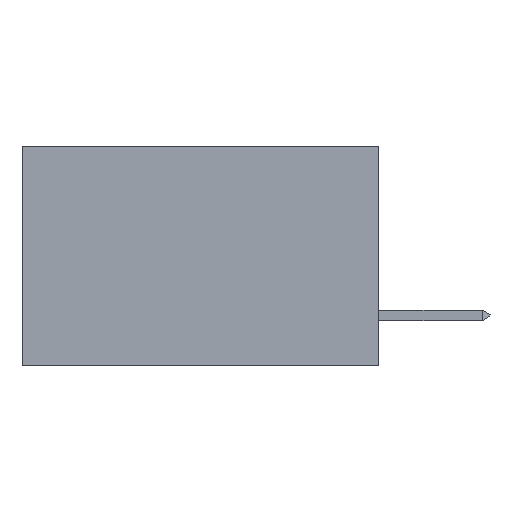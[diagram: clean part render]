
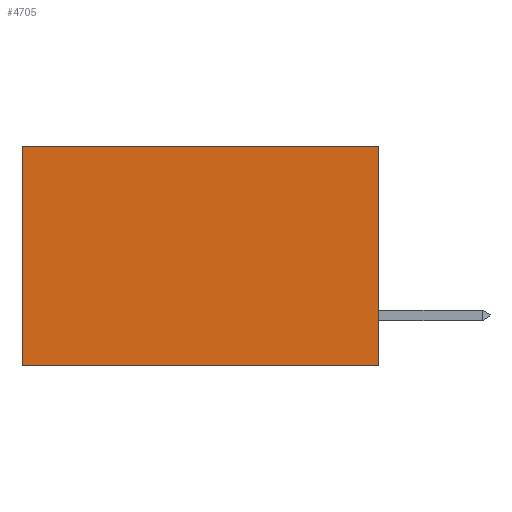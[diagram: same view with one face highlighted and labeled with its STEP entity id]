
A CAD part, left-side view. The second image highlights one B-rep face of the part: STEP entity #4705.
In plain terms, the highlighted planar face has unit normal (-1, 0, 0).
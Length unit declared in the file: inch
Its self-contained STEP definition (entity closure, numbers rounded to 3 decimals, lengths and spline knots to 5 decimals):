
#309 = PLANE ( 'NONE',  #9736 ) ;
#553 = CARTESIAN_POINT ( 'NONE',  ( 0.2615, 0.6, -0.37 ) ) ;
#567 = LINE ( 'NONE', #10985, #5831 ) ;
#1402 = VERTEX_POINT ( 'NONE', #7710 ) ;
#2370 = VECTOR ( 'NONE', #8470, 39.37008 ) ;
#2410 = CARTESIAN_POINT ( 'NONE',  ( 0.2615, 0.6, 0. ) ) ;
#2678 = ORIENTED_EDGE ( 'NONE', *, *, #9156, .T. ) ;
#3394 = EDGE_LOOP ( 'NONE', ( #2678, #6692, #9262, #9863 ) ) ;
#3428 = CARTESIAN_POINT ( 'NONE',  ( 0.2615, 0., -0.37 ) ) ;
#4469 = CARTESIAN_POINT ( 'NONE',  ( 0.2615, 0., -0.37 ) ) ;
#4680 = DIRECTION ( 'NONE',  ( 0., 0., -1. ) ) ;
#4705 = ADVANCED_FACE ( 'NONE', ( #9632 ), #309, .F. ) ;
#4862 = VERTEX_POINT ( 'NONE', #5991 ) ;
#4939 = EDGE_CURVE ( 'NONE', #1402, #5220, #567, .T. ) ;
#5204 = VERTEX_POINT ( 'NONE', #3428 ) ;
#5220 = VERTEX_POINT ( 'NONE', #2410 ) ;
#5831 = VECTOR ( 'NONE', #8918, 39.37008 ) ;
#5991 = CARTESIAN_POINT ( 'NONE',  ( 0.2615, 0.6, -0.37 ) ) ;
#6692 = ORIENTED_EDGE ( 'NONE', *, *, #8149, .F. ) ;
#7191 = VECTOR ( 'NONE', #4680, 39.37008 ) ;
#7710 = CARTESIAN_POINT ( 'NONE',  ( 0.2615, 0., 0. ) ) ;
#8149 = EDGE_CURVE ( 'NONE', #5204, #4862, #12806, .T. ) ;
#8201 = CARTESIAN_POINT ( 'NONE',  ( 0.2615, 0., -0.37 ) ) ;
#8470 = DIRECTION ( 'NONE',  ( 0., 1., 0. ) ) ;
#8576 = DIRECTION ( 'NONE',  ( 0., 0., -1. ) ) ;
#8830 = LINE ( 'NONE', #553, #7191 ) ;
#8918 = DIRECTION ( 'NONE',  ( 0., 1., 0. ) ) ;
#9156 = EDGE_CURVE ( 'NONE', #5220, #4862, #8830, .T. ) ;
#9262 = ORIENTED_EDGE ( 'NONE', *, *, #9331, .F. ) ;
#9331 = EDGE_CURVE ( 'NONE', #1402, #5204, #10266, .T. ) ;
#9487 = CARTESIAN_POINT ( 'NONE',  ( 0.2615, 0., -0.37 ) ) ;
#9632 = FACE_OUTER_BOUND ( 'NONE', #3394, .T. ) ;
#9736 = AXIS2_PLACEMENT_3D ( 'NONE', #9487, #10520, #8576 ) ;
#9863 = ORIENTED_EDGE ( 'NONE', *, *, #4939, .T. ) ;
#10266 = LINE ( 'NONE', #8201, #12008 ) ;
#10520 = DIRECTION ( 'NONE',  ( 1., 0., 0. ) ) ;
#10985 = CARTESIAN_POINT ( 'NONE',  ( 0.2615, 0., 0. ) ) ;
#12008 = VECTOR ( 'NONE', #13371, 39.37008 ) ;
#12806 = LINE ( 'NONE', #4469, #2370 ) ;
#13371 = DIRECTION ( 'NONE',  ( 0., 0., -1. ) ) ;
